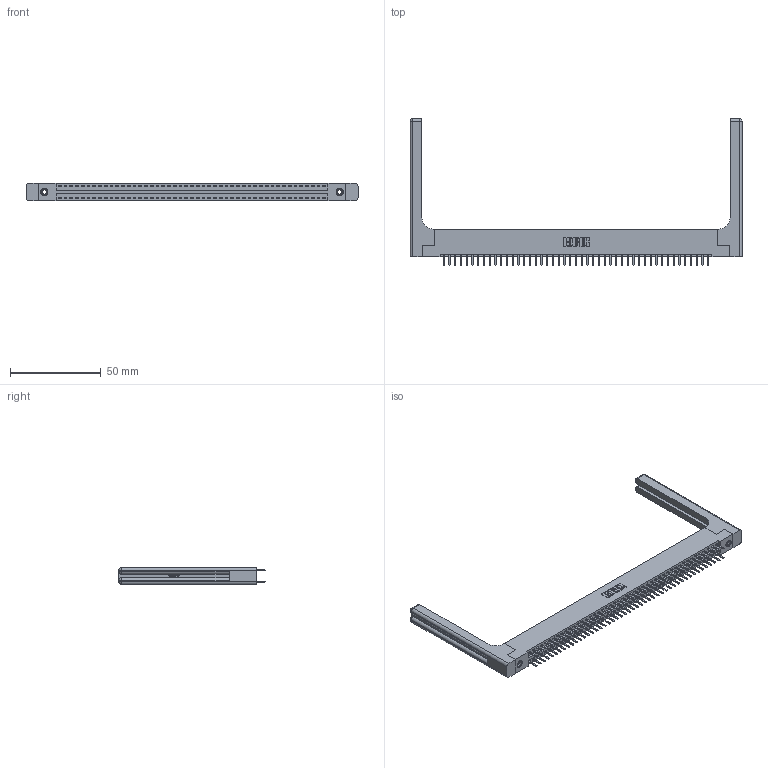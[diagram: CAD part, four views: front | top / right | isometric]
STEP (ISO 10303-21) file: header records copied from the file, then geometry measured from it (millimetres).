
FILE_DESCRIPTION (( 'STEP AP203' ), '1' );
FILE_NAME ('346-094-520-258.STEP', '2022-05-26T09:24:12', ( '' ), ( '' ), 'SwSTEP 2.0', 'SolidWorks 2020', '' );
FILE_SCHEMA (( 'CONFIG_CONTROL_DESIGN' ));
Length unit declared in the file: inch
Products named in the file (5): 345-250-001_345-250-001-102; 346 Part_Flush Mounting Lugs - 0.156 Dia-TH; 346-220-058_345-220-058; 346-094-520-258; 345-292-001_345-293-120
Assembly tree (99 placements, depth 2):
  346-094-520-258
    346 Part_Flush Mounting Lugs - 0.156 Dia-TH
    345-292-001_345-293-120  x94
    345-250-001_345-250-001-102  x2
    346-220-058_345-220-058  x2
Bounding box: 183.29 x 80.98 x 9.4 mm (x, y, z)
Volume: 25346.4 mm3; surface area: 29528 mm2
Topology: 99 solids, 99 shells, 5656 faces, 16353 edges, 10630 vertices
Faces by surface type: plane 3716, cylinder 1880, bspline 36, cone 12, sphere 8, torus 4
Entity records: 35712 total; most frequent: CARTESIAN_POINT 6903, ORIENTED_EDGE 5620, DIRECTION 5054, EDGE_CURVE 2810, LINE 2394, VECTOR 2394, VERTEX_POINT 1862, AXIS2_PLACEMENT_3D 1330
